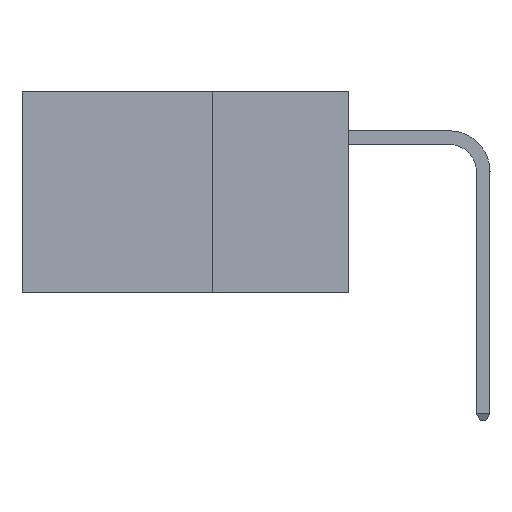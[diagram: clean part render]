
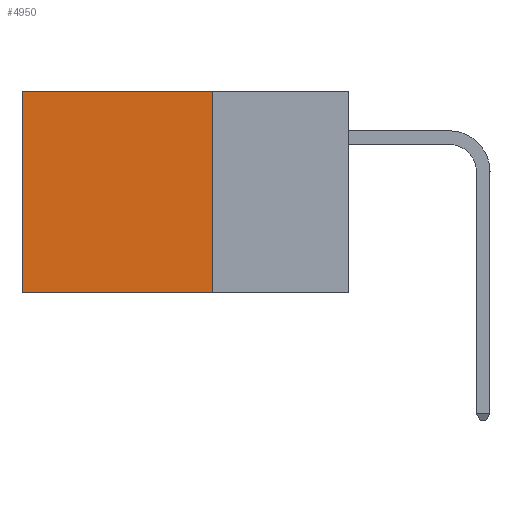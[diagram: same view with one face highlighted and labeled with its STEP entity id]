
A CAD part, left-side view. The second image highlights one B-rep face of the part: STEP entity #4950.
In plain terms, the highlighted planar face has unit normal (-1, 0, 0).
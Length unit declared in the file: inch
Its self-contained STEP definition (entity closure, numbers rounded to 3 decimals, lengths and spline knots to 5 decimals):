
#428 = ORIENTED_EDGE ( 'NONE', *, *, #11505, .F. ) ;
#522 = LINE ( 'NONE', #10878, #11294 ) ;
#649 = CARTESIAN_POINT ( 'NONE',  ( 0.2875, 0.25, -0.37 ) ) ;
#1202 = ORIENTED_EDGE ( 'NONE', *, *, #14339, .T. ) ;
#1204 = AXIS2_PLACEMENT_3D ( 'NONE', #5224, #7741, #6569 ) ;
#2411 = EDGE_LOOP ( 'NONE', ( #5054, #428, #12475, #1202 ) ) ;
#2685 = DIRECTION ( 'NONE',  ( 0., 1., 0. ) ) ;
#2766 = EDGE_CURVE ( 'NONE', #3216, #11274, #14026, .T. ) ;
#3216 = VERTEX_POINT ( 'NONE', #6886 ) ;
#3876 = VECTOR ( 'NONE', #9548, 39.37008 ) ;
#4750 = CARTESIAN_POINT ( 'NONE',  ( 0.2875, 0.6, -0.37 ) ) ;
#4950 = ADVANCED_FACE ( 'NONE', ( #5243 ), #5272, .F. ) ;
#5054 = ORIENTED_EDGE ( 'NONE', *, *, #13195, .T. ) ;
#5224 = CARTESIAN_POINT ( 'NONE',  ( 0.2875, 0.25, 0. ) ) ;
#5243 = FACE_OUTER_BOUND ( 'NONE', #2411, .T. ) ;
#5272 = PLANE ( 'NONE',  #1204 ) ;
#5312 = VECTOR ( 'NONE', #7274, 39.37008 ) ;
#5537 = DIRECTION ( 'NONE',  ( 0., 0., -1. ) ) ;
#5835 = CARTESIAN_POINT ( 'NONE',  ( 0.2875, 0.6, 0. ) ) ;
#6569 = DIRECTION ( 'NONE',  ( 0., 0., -1. ) ) ;
#6694 = VECTOR ( 'NONE', #2685, 39.37008 ) ;
#6728 = CARTESIAN_POINT ( 'NONE',  ( 0.2875, 0.25, 0. ) ) ;
#6819 = LINE ( 'NONE', #13920, #3876 ) ;
#6886 = CARTESIAN_POINT ( 'NONE',  ( 0.2875, 0.25, 0. ) ) ;
#7274 = DIRECTION ( 'NONE',  ( 0., 0., -1. ) ) ;
#7366 = LINE ( 'NONE', #12554, #6694 ) ;
#7741 = DIRECTION ( 'NONE',  ( 1., 0., 0. ) ) ;
#8638 = VERTEX_POINT ( 'NONE', #5835 ) ;
#9548 = DIRECTION ( 'NONE',  ( 0., 1., 0. ) ) ;
#10878 = CARTESIAN_POINT ( 'NONE',  ( 0.2875, 0.6, 0. ) ) ;
#11274 = VERTEX_POINT ( 'NONE', #649 ) ;
#11294 = VECTOR ( 'NONE', #5537, 39.37008 ) ;
#11505 = EDGE_CURVE ( 'NONE', #11274, #12095, #7366, .T. ) ;
#12095 = VERTEX_POINT ( 'NONE', #4750 ) ;
#12475 = ORIENTED_EDGE ( 'NONE', *, *, #2766, .F. ) ;
#12554 = CARTESIAN_POINT ( 'NONE',  ( 0.2875, 0.25, -0.37 ) ) ;
#13195 = EDGE_CURVE ( 'NONE', #8638, #12095, #522, .T. ) ;
#13920 = CARTESIAN_POINT ( 'NONE',  ( 0.2875, 0.25, 0. ) ) ;
#14026 = LINE ( 'NONE', #6728, #5312 ) ;
#14339 = EDGE_CURVE ( 'NONE', #3216, #8638, #6819, .T. ) ;
